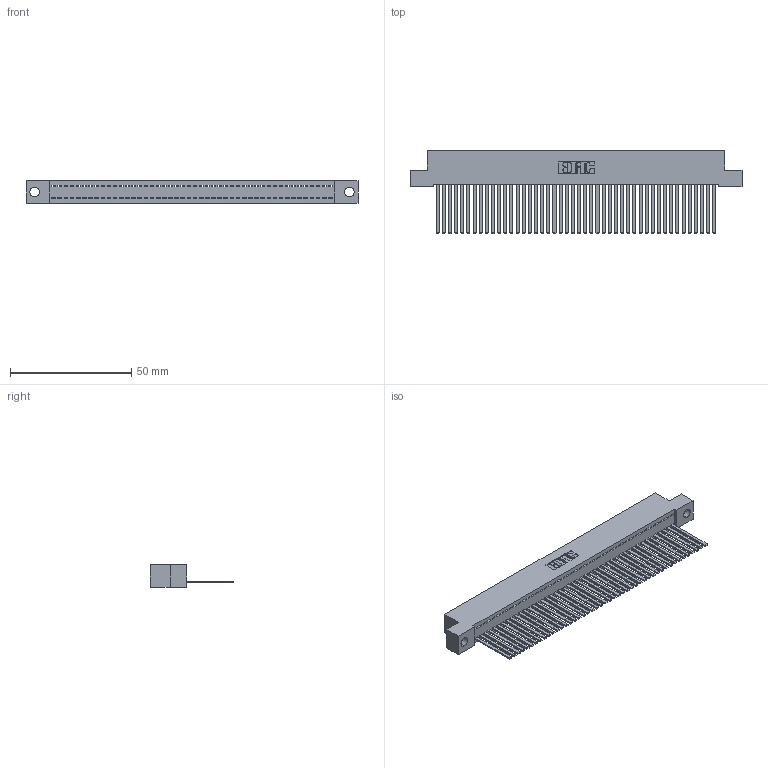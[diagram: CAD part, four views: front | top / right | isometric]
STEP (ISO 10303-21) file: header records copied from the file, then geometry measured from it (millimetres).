
FILE_DESCRIPTION (( 'STEP AP203' ), '1' );
FILE_NAME ('342-046-544-104.STEP', '2019-10-02T20:45:58', ( '' ), ( '' ), 'SwSTEP 2.0', 'SolidWorks 2016', '' );
FILE_SCHEMA (( 'CONFIG_CONTROL_DESIGN' ));
Length unit declared in the file: inch
Products named in the file (3): 342 Part_.156 TH; 345-292-001_345-293-144; 342-046-544-104
Assembly tree (47 placements, depth 2):
  342-046-544-104
    342 Part_.156 TH
    345-292-001_345-293-144  x46
Bounding box: 137.16 x 34.3 x 9.4 mm (x, y, z)
Volume: 12486.6 mm3; surface area: 19745.8 mm2
Topology: 47 solids, 47 shells, 2502 faces, 7567 edges, 4982 vertices
Faces by surface type: plane 1814, cylinder 688
Entity records: 27291 total; most frequent: CARTESIAN_POINT 4712, ORIENTED_EDGE 4694, DIRECTION 3963, EDGE_CURVE 2347, LINE 2223, VECTOR 2223, VERTEX_POINT 1562, AXIS2_PLACEMENT_3D 870
